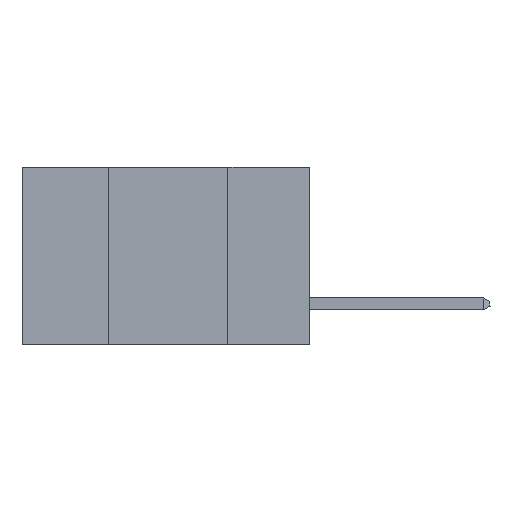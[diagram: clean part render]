
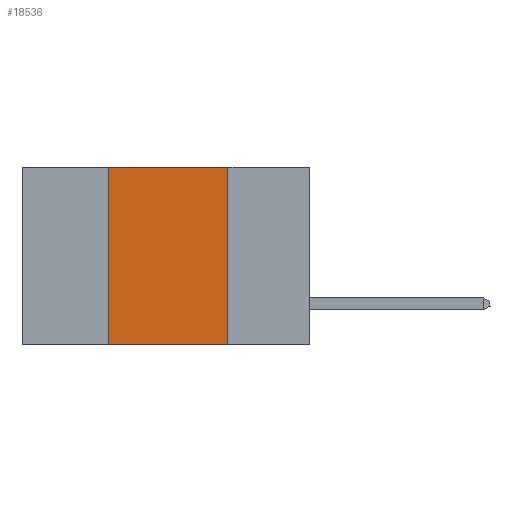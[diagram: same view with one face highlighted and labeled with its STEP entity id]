
A CAD part, left-side view. The second image highlights one B-rep face of the part: STEP entity #18536.
In plain terms, the highlighted planar face has unit normal (-1, 0, 0).
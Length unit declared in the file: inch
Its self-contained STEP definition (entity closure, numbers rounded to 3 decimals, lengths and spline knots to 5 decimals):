
#723 = PLANE ( 'NONE',  #28017 ) ;
#1525 = CARTESIAN_POINT ( 'NONE',  ( 0., 0.6, -0.37 ) ) ;
#2792 = VERTEX_POINT ( 'NONE', #33230 ) ;
#4298 = DIRECTION ( 'NONE',  ( 1., 0., 0. ) ) ;
#6628 = DIRECTION ( 'NONE',  ( 0., 0., -1. ) ) ;
#8449 = EDGE_CURVE ( 'NONE', #30514, #36085, #10172, .T. ) ;
#8719 = ORIENTED_EDGE ( 'NONE', *, *, #13990, .T. ) ;
#8832 = VERTEX_POINT ( 'NONE', #23204 ) ;
#9142 = CARTESIAN_POINT ( 'NONE',  ( 0., 0.42, 0. ) ) ;
#9657 = VECTOR ( 'NONE', #34832, 39.37008 ) ;
#10172 = LINE ( 'NONE', #45659, #9657 ) ;
#10490 = CARTESIAN_POINT ( 'NONE',  ( 0., 0.42, -0.37 ) ) ;
#13990 = EDGE_CURVE ( 'NONE', #30514, #2792, #23824, .T. ) ;
#18451 = EDGE_CURVE ( 'NONE', #8832, #2792, #38267, .T. ) ;
#18536 = ADVANCED_FACE ( 'NONE', ( #26181 ), #723, .F. ) ;
#19202 = ORIENTED_EDGE ( 'NONE', *, *, #33674, .F. ) ;
#19550 = VECTOR ( 'NONE', #6628, 39.37008 ) ;
#23204 = CARTESIAN_POINT ( 'NONE',  ( 0., 0.17, 0. ) ) ;
#23824 = LINE ( 'NONE', #1525, #40428 ) ;
#25555 = CARTESIAN_POINT ( 'NONE',  ( 0., 0.6, 0. ) ) ;
#26181 = FACE_OUTER_BOUND ( 'NONE', #35993, .T. ) ;
#28017 = AXIS2_PLACEMENT_3D ( 'NONE', #25555, #4298, #36398 ) ;
#29131 = LINE ( 'NONE', #39475, #35819 ) ;
#30062 = DIRECTION ( 'NONE',  ( 0., -1., 0. ) ) ;
#30491 = DIRECTION ( 'NONE',  ( 0., -1., 0. ) ) ;
#30514 = VERTEX_POINT ( 'NONE', #10490 ) ;
#30936 = ORIENTED_EDGE ( 'NONE', *, *, #8449, .F. ) ;
#33230 = CARTESIAN_POINT ( 'NONE',  ( 0., 0.17, -0.37 ) ) ;
#33674 = EDGE_CURVE ( 'NONE', #36085, #8832, #29131, .T. ) ;
#34131 = ORIENTED_EDGE ( 'NONE', *, *, #18451, .F. ) ;
#34832 = DIRECTION ( 'NONE',  ( 0., 0., 1. ) ) ;
#35819 = VECTOR ( 'NONE', #30062, 39.37008 ) ;
#35993 = EDGE_LOOP ( 'NONE', ( #34131, #19202, #30936, #8719 ) ) ;
#36085 = VERTEX_POINT ( 'NONE', #9142 ) ;
#36398 = DIRECTION ( 'NONE',  ( 0., 0., -1. ) ) ;
#38267 = LINE ( 'NONE', #41521, #19550 ) ;
#39475 = CARTESIAN_POINT ( 'NONE',  ( 0., 0.6, 0. ) ) ;
#40428 = VECTOR ( 'NONE', #30491, 39.37008 ) ;
#41521 = CARTESIAN_POINT ( 'NONE',  ( 0., 0.17, 0. ) ) ;
#45659 = CARTESIAN_POINT ( 'NONE',  ( 0., 0.42, 0. ) ) ;
